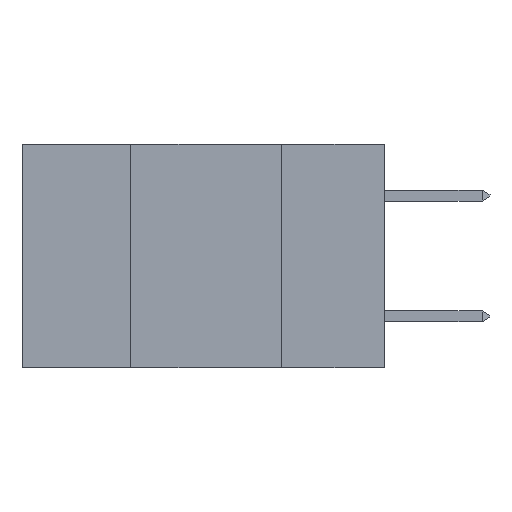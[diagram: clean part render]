
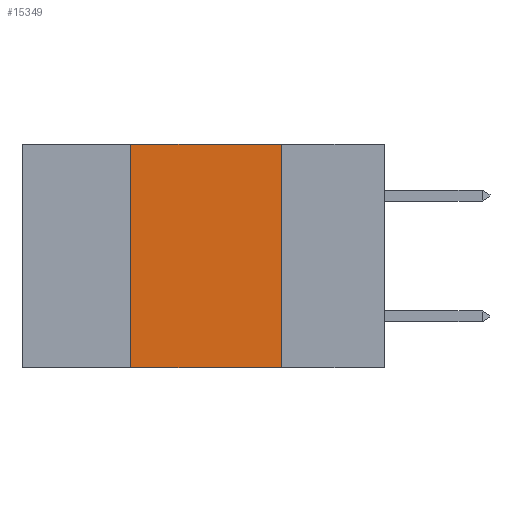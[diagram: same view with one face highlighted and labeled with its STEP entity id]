
A CAD part, left-side view. The second image highlights one B-rep face of the part: STEP entity #15349.
In plain terms, the highlighted planar face has unit normal (-1, 0, 0).
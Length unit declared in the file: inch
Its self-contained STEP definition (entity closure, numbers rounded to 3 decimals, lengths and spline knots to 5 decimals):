
#2319 = VECTOR ( 'NONE', #23089, 39.37008 ) ;
#6541 = PLANE ( 'NONE',  #18483 ) ;
#6737 = LINE ( 'NONE', #24513, #23351 ) ;
#6837 = ORIENTED_EDGE ( 'NONE', *, *, #16206, .T. ) ;
#7284 = CARTESIAN_POINT ( 'NONE',  ( 0., 0.17, 0. ) ) ;
#8550 = VERTEX_POINT ( 'NONE', #24542 ) ;
#9610 = VECTOR ( 'NONE', #11117, 39.37008 ) ;
#11117 = DIRECTION ( 'NONE',  ( 0., -1., 0. ) ) ;
#11130 = FACE_OUTER_BOUND ( 'NONE', #13615, .T. ) ;
#11534 = ORIENTED_EDGE ( 'NONE', *, *, #12157, .F. ) ;
#12157 = EDGE_CURVE ( 'NONE', #24598, #18795, #6737, .T. ) ;
#12231 = CARTESIAN_POINT ( 'NONE',  ( 0., 0.42, 0. ) ) ;
#13615 = EDGE_LOOP ( 'NONE', ( #20954, #11534, #23771, #6837 ) ) ;
#14215 = DIRECTION ( 'NONE',  ( 0., 0., -1. ) ) ;
#14946 = CARTESIAN_POINT ( 'NONE',  ( 0., 0.42, 0. ) ) ;
#15349 = ADVANCED_FACE ( 'NONE', ( #11130 ), #6541, .F. ) ;
#15464 = VERTEX_POINT ( 'NONE', #18653 ) ;
#15703 = CARTESIAN_POINT ( 'NONE',  ( 0., 0.17, 0. ) ) ;
#16206 = EDGE_CURVE ( 'NONE', #8550, #15464, #19727, .T. ) ;
#16276 = VECTOR ( 'NONE', #17707, 39.37008 ) ;
#17707 = DIRECTION ( 'NONE',  ( 0., 0., -1. ) ) ;
#18483 = AXIS2_PLACEMENT_3D ( 'NONE', #19901, #23727, #14215 ) ;
#18653 = CARTESIAN_POINT ( 'NONE',  ( 0., 0.17, -0.37 ) ) ;
#18795 = VERTEX_POINT ( 'NONE', #7284 ) ;
#19263 = EDGE_CURVE ( 'NONE', #18795, #15464, #21332, .T. ) ;
#19727 = LINE ( 'NONE', #20950, #9610 ) ;
#19901 = CARTESIAN_POINT ( 'NONE',  ( 0., 0.6, 0. ) ) ;
#20950 = CARTESIAN_POINT ( 'NONE',  ( 0., 0.6, -0.37 ) ) ;
#20954 = ORIENTED_EDGE ( 'NONE', *, *, #19263, .F. ) ;
#20969 = EDGE_CURVE ( 'NONE', #8550, #24598, #21685, .T. ) ;
#21332 = LINE ( 'NONE', #15703, #16276 ) ;
#21685 = LINE ( 'NONE', #14946, #2319 ) ;
#22603 = DIRECTION ( 'NONE',  ( 0., -1., 0. ) ) ;
#23089 = DIRECTION ( 'NONE',  ( 0., 0., 1. ) ) ;
#23351 = VECTOR ( 'NONE', #22603, 39.37008 ) ;
#23727 = DIRECTION ( 'NONE',  ( 1., 0., 0. ) ) ;
#23771 = ORIENTED_EDGE ( 'NONE', *, *, #20969, .F. ) ;
#24513 = CARTESIAN_POINT ( 'NONE',  ( 0., 0.6, 0. ) ) ;
#24542 = CARTESIAN_POINT ( 'NONE',  ( 0., 0.42, -0.37 ) ) ;
#24598 = VERTEX_POINT ( 'NONE', #12231 ) ;
